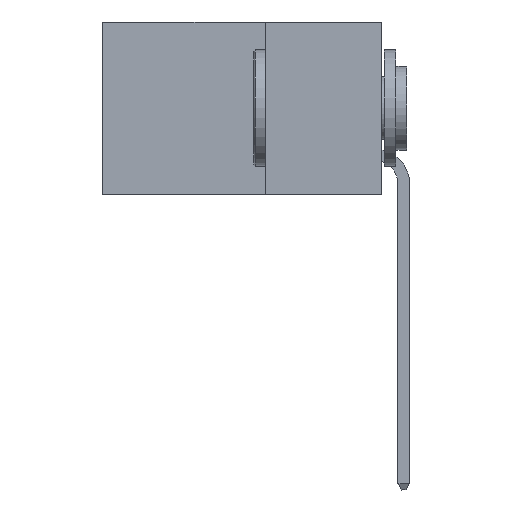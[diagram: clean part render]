
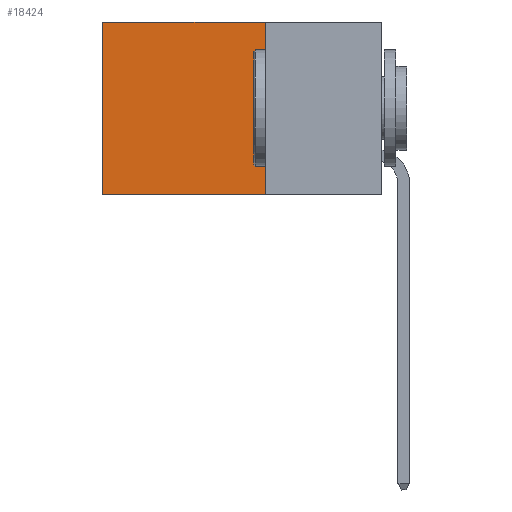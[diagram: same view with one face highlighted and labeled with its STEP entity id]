
A CAD part, left-side view. The second image highlights one B-rep face of the part: STEP entity #18424.
In plain terms, the highlighted planar face has unit normal (-1, 0, 0).
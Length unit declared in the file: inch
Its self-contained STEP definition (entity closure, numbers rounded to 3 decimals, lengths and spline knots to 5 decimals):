
#1186 = DIRECTION ( 'NONE',  ( 0., 1., 0. ) ) ;
#1795 = VECTOR ( 'NONE', #8498, 39.37008 ) ;
#2900 = VERTEX_POINT ( 'NONE', #30170 ) ;
#4052 = FACE_OUTER_BOUND ( 'NONE', #29812, .T. ) ;
#5199 = VERTEX_POINT ( 'NONE', #11751 ) ;
#5505 = CARTESIAN_POINT ( 'NONE',  ( 0.2875, 0.6, 0. ) ) ;
#5798 = PLANE ( 'NONE',  #35186 ) ;
#7363 = CARTESIAN_POINT ( 'NONE',  ( 0.2875, 0.25, -0.37 ) ) ;
#8498 = DIRECTION ( 'NONE',  ( 0., 0., -1. ) ) ;
#9409 = LINE ( 'NONE', #18723, #33545 ) ;
#10161 = LINE ( 'NONE', #7363, #32462 ) ;
#10311 = DIRECTION ( 'NONE',  ( 0., 1., 0. ) ) ;
#11751 = CARTESIAN_POINT ( 'NONE',  ( 0.2875, 0.25, -0.37 ) ) ;
#11832 = EDGE_CURVE ( 'NONE', #2900, #5199, #14003, .T. ) ;
#14003 = LINE ( 'NONE', #14709, #21690 ) ;
#14594 = CARTESIAN_POINT ( 'NONE',  ( 0.2875, 0.25, 0. ) ) ;
#14709 = CARTESIAN_POINT ( 'NONE',  ( 0.2875, 0.25, 0. ) ) ;
#16146 = ORIENTED_EDGE ( 'NONE', *, *, #24483, .F. ) ;
#17468 = DIRECTION ( 'NONE',  ( 0., 0., -1. ) ) ;
#18424 = ADVANCED_FACE ( 'NONE', ( #4052 ), #5798, .F. ) ;
#18723 = CARTESIAN_POINT ( 'NONE',  ( 0.2875, 0.25, 0. ) ) ;
#19203 = LINE ( 'NONE', #5505, #1795 ) ;
#19228 = ORIENTED_EDGE ( 'NONE', *, *, #20709, .T. ) ;
#20709 = EDGE_CURVE ( 'NONE', #2900, #29887, #9409, .T. ) ;
#21690 = VECTOR ( 'NONE', #23461, 39.37008 ) ;
#22835 = EDGE_CURVE ( 'NONE', #29887, #32274, #19203, .T. ) ;
#23259 = CARTESIAN_POINT ( 'NONE',  ( 0.2875, 0.6, -0.37 ) ) ;
#23461 = DIRECTION ( 'NONE',  ( 0., 0., -1. ) ) ;
#24483 = EDGE_CURVE ( 'NONE', #5199, #32274, #10161, .T. ) ;
#27957 = CARTESIAN_POINT ( 'NONE',  ( 0.2875, 0.6, 0. ) ) ;
#29617 = ORIENTED_EDGE ( 'NONE', *, *, #11832, .F. ) ;
#29812 = EDGE_LOOP ( 'NONE', ( #30384, #16146, #29617, #19228 ) ) ;
#29887 = VERTEX_POINT ( 'NONE', #27957 ) ;
#30170 = CARTESIAN_POINT ( 'NONE',  ( 0.2875, 0.25, 0. ) ) ;
#30384 = ORIENTED_EDGE ( 'NONE', *, *, #22835, .T. ) ;
#32274 = VERTEX_POINT ( 'NONE', #23259 ) ;
#32462 = VECTOR ( 'NONE', #10311, 39.37008 ) ;
#33545 = VECTOR ( 'NONE', #1186, 39.37008 ) ;
#34989 = DIRECTION ( 'NONE',  ( 1., 0., 0. ) ) ;
#35186 = AXIS2_PLACEMENT_3D ( 'NONE', #14594, #34989, #17468 ) ;
